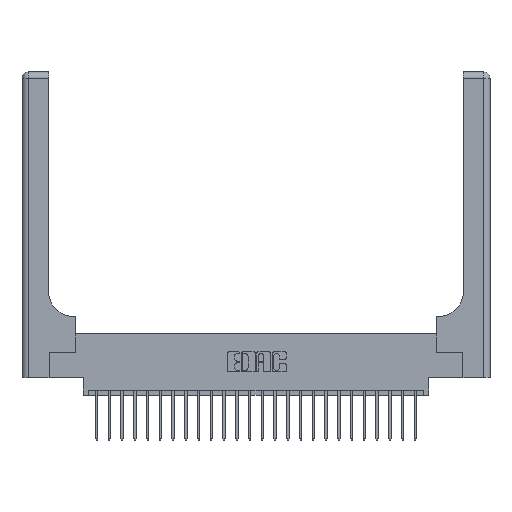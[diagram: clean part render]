
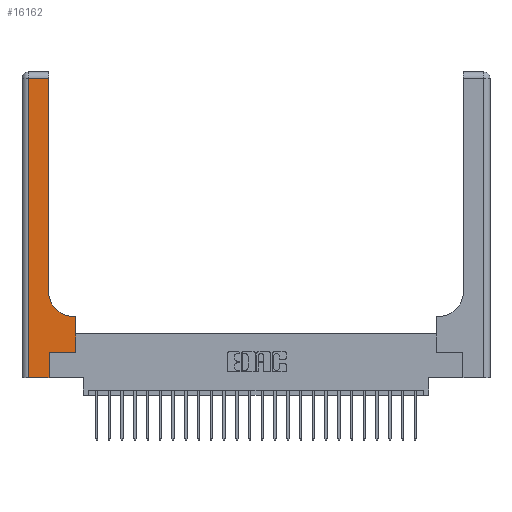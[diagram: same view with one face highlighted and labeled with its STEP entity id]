
A CAD part, top view. The second image highlights one B-rep face of the part: STEP entity #16162.
In plain terms, the highlighted planar face has unit normal (0, 0, 1).
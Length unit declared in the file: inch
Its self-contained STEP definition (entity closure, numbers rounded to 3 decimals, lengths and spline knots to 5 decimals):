
#284 = ORIENTED_EDGE ( 'NONE', *, *, #4571, .T. ) ;
#477 = DIRECTION ( 'NONE',  ( 0., 1., 0. ) ) ;
#529 = CIRCLE ( 'NONE', #23951, 0.25 ) ;
#650 = CARTESIAN_POINT ( 'NONE',  ( 0.06, 0., 0.37 ) ) ;
#1835 = CARTESIAN_POINT ( 'NONE',  ( 0.26, 0.6, 0.37 ) ) ;
#2197 = CARTESIAN_POINT ( 'NONE',  ( 0.265, 0.25, 0.37 ) ) ;
#2213 = VECTOR ( 'NONE', #22079, 39.37008 ) ;
#3016 = VERTEX_POINT ( 'NONE', #7233 ) ;
#3455 = EDGE_CURVE ( 'NONE', #17525, #17911, #19779, .T. ) ;
#3692 = CARTESIAN_POINT ( 'NONE',  ( 0., 3., 0.37 ) ) ;
#3964 = LINE ( 'NONE', #24391, #14105 ) ;
#4480 = DIRECTION ( 'NONE',  ( 0., 0., -1. ) ) ;
#4571 = EDGE_CURVE ( 'NONE', #14738, #17525, #7297, .T. ) ;
#5160 = AXIS2_PLACEMENT_3D ( 'NONE', #3692, #20736, #9443 ) ;
#5485 = EDGE_CURVE ( 'NONE', #9194, #14738, #3964, .T. ) ;
#5980 = VECTOR ( 'NONE', #13922, 39.37008 ) ;
#6307 = VECTOR ( 'NONE', #13186, 39.37008 ) ;
#6690 = VERTEX_POINT ( 'NONE', #15613 ) ;
#7013 = CARTESIAN_POINT ( 'NONE',  ( 0., 0., 0.37 ) ) ;
#7233 = CARTESIAN_POINT ( 'NONE',  ( 0.26, 2.94, 0.37 ) ) ;
#7297 = LINE ( 'NONE', #7013, #2213 ) ;
#7378 = PLANE ( 'NONE',  #5160 ) ;
#7792 = VERTEX_POINT ( 'NONE', #22012 ) ;
#8658 = VECTOR ( 'NONE', #19281, 39.37008 ) ;
#9026 = VECTOR ( 'NONE', #23882, 39.37008 ) ;
#9157 = CARTESIAN_POINT ( 'NONE',  ( 0.528, 0.6, 0.37 ) ) ;
#9194 = VERTEX_POINT ( 'NONE', #22369 ) ;
#9240 = ORIENTED_EDGE ( 'NONE', *, *, #17589, .T. ) ;
#9372 = ORIENTED_EDGE ( 'NONE', *, *, #15786, .T. ) ;
#9443 = DIRECTION ( 'NONE',  ( -1., 0., 0. ) ) ;
#9482 = ORIENTED_EDGE ( 'NONE', *, *, #3455, .T. ) ;
#11463 = CARTESIAN_POINT ( 'NONE',  ( 0.265, 0.25, 0.37 ) ) ;
#12126 = EDGE_LOOP ( 'NONE', ( #21770, #12384, #14931, #284, #9482, #9372, #24382, #19336, #9240 ) ) ;
#12384 = ORIENTED_EDGE ( 'NONE', *, *, #12898, .T. ) ;
#12607 = EDGE_CURVE ( 'NONE', #13210, #6690, #20773, .T. ) ;
#12690 = CARTESIAN_POINT ( 'NONE',  ( 0.528, 0.25, 0.37 ) ) ;
#12831 = EDGE_CURVE ( 'NONE', #7792, #3016, #22202, .T. ) ;
#12898 = EDGE_CURVE ( 'NONE', #3016, #9194, #15481, .T. ) ;
#13186 = DIRECTION ( 'NONE',  ( -1., 0., 0. ) ) ;
#13210 = VERTEX_POINT ( 'NONE', #9157 ) ;
#13720 = LINE ( 'NONE', #2197, #8658 ) ;
#13922 = DIRECTION ( 'NONE',  ( -1., 0., 0. ) ) ;
#14003 = CARTESIAN_POINT ( 'NONE',  ( 0., 2.94, 0.37 ) ) ;
#14105 = VECTOR ( 'NONE', #15094, 39.37008 ) ;
#14361 = DIRECTION ( 'NONE',  ( 0., 1., 0. ) ) ;
#14738 = VERTEX_POINT ( 'NONE', #650 ) ;
#14931 = ORIENTED_EDGE ( 'NONE', *, *, #5485, .T. ) ;
#15094 = DIRECTION ( 'NONE',  ( 0., -1., 0. ) ) ;
#15457 = FACE_OUTER_BOUND ( 'NONE', #12126, .T. ) ;
#15481 = LINE ( 'NONE', #14003, #5980 ) ;
#15613 = CARTESIAN_POINT ( 'NONE',  ( 0.51, 0.6, 0.37 ) ) ;
#15786 = EDGE_CURVE ( 'NONE', #17911, #23792, #13720, .T. ) ;
#15876 = CARTESIAN_POINT ( 'NONE',  ( 0.51, 0.85, 0.37 ) ) ;
#16162 = ADVANCED_FACE ( 'NONE', ( #15457 ), #7378, .F. ) ;
#16431 = CARTESIAN_POINT ( 'NONE',  ( 0.528, 0.25, 0.37 ) ) ;
#17525 = VERTEX_POINT ( 'NONE', #19236 ) ;
#17589 = EDGE_CURVE ( 'NONE', #6690, #7792, #529, .T. ) ;
#17754 = DIRECTION ( 'NONE',  ( 1., 0., 0. ) ) ;
#17911 = VERTEX_POINT ( 'NONE', #11463 ) ;
#19236 = CARTESIAN_POINT ( 'NONE',  ( 0.265, 0., 0.37 ) ) ;
#19281 = DIRECTION ( 'NONE',  ( 1., 0., 0. ) ) ;
#19336 = ORIENTED_EDGE ( 'NONE', *, *, #12607, .T. ) ;
#19679 = LINE ( 'NONE', #12690, #9026 ) ;
#19779 = LINE ( 'NONE', #23645, #24109 ) ;
#20736 = DIRECTION ( 'NONE',  ( 0., 0., -1. ) ) ;
#20773 = LINE ( 'NONE', #1835, #6307 ) ;
#21041 = VECTOR ( 'NONE', #477, 39.37008 ) ;
#21344 = EDGE_CURVE ( 'NONE', #23792, #13210, #19679, .T. ) ;
#21770 = ORIENTED_EDGE ( 'NONE', *, *, #12831, .T. ) ;
#22012 = CARTESIAN_POINT ( 'NONE',  ( 0.26, 0.85, 0.37 ) ) ;
#22079 = DIRECTION ( 'NONE',  ( 1., 0., 0. ) ) ;
#22202 = LINE ( 'NONE', #23148, #21041 ) ;
#22369 = CARTESIAN_POINT ( 'NONE',  ( 0.06, 2.94, 0.37 ) ) ;
#23148 = CARTESIAN_POINT ( 'NONE',  ( 0.26, 3., 0.37 ) ) ;
#23645 = CARTESIAN_POINT ( 'NONE',  ( 0.265, 0., 0.37 ) ) ;
#23792 = VERTEX_POINT ( 'NONE', #16431 ) ;
#23882 = DIRECTION ( 'NONE',  ( 0., 1., 0. ) ) ;
#23951 = AXIS2_PLACEMENT_3D ( 'NONE', #15876, #4480, #17754 ) ;
#24109 = VECTOR ( 'NONE', #14361, 39.37008 ) ;
#24382 = ORIENTED_EDGE ( 'NONE', *, *, #21344, .T. ) ;
#24391 = CARTESIAN_POINT ( 'NONE',  ( 0.06, 3., 0.37 ) ) ;
